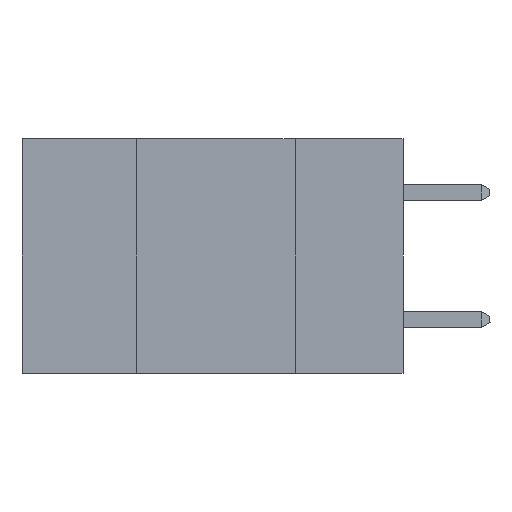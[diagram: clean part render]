
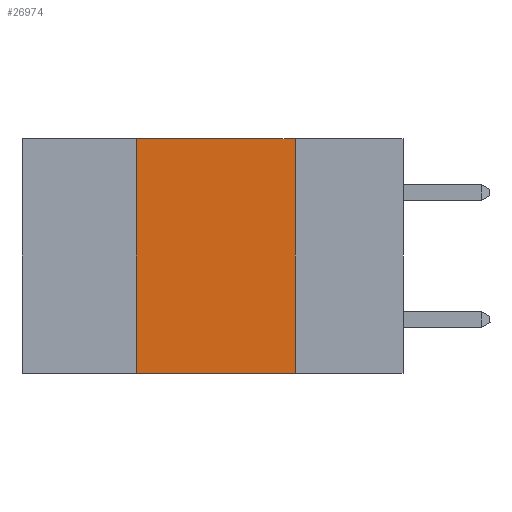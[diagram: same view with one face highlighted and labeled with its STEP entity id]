
A CAD part, left-side view. The second image highlights one B-rep face of the part: STEP entity #26974.
In plain terms, the highlighted planar face has unit normal (-1, 0, 0).
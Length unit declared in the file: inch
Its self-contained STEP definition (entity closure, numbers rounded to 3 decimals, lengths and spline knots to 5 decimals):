
#335 = CARTESIAN_POINT ( 'NONE',  ( 0., 0.6, -0.37 ) ) ;
#423 = EDGE_LOOP ( 'NONE', ( #12382, #18874, #16290, #22187 ) ) ;
#1531 = CARTESIAN_POINT ( 'NONE',  ( 0., 0.42, 0. ) ) ;
#4603 = CARTESIAN_POINT ( 'NONE',  ( 0., 0.17, -0.37 ) ) ;
#5061 = VERTEX_POINT ( 'NONE', #4603 ) ;
#5590 = EDGE_CURVE ( 'NONE', #26018, #29388, #32946, .T. ) ;
#6365 = PLANE ( 'NONE',  #26450 ) ;
#6553 = DIRECTION ( 'NONE',  ( 0., 0., 1. ) ) ;
#7317 = VECTOR ( 'NONE', #6553, 39.37008 ) ;
#8792 = FACE_OUTER_BOUND ( 'NONE', #423, .T. ) ;
#8803 = CARTESIAN_POINT ( 'NONE',  ( 0., 0.42, 0. ) ) ;
#9530 = DIRECTION ( 'NONE',  ( 0., -1., 0. ) ) ;
#9586 = EDGE_CURVE ( 'NONE', #29388, #25753, #22335, .T. ) ;
#10875 = LINE ( 'NONE', #335, #19131 ) ;
#11165 = VECTOR ( 'NONE', #9530, 39.37008 ) ;
#11464 = CARTESIAN_POINT ( 'NONE',  ( 0., 0.6, 0. ) ) ;
#12179 = LINE ( 'NONE', #23573, #29580 ) ;
#12382 = ORIENTED_EDGE ( 'NONE', *, *, #25512, .F. ) ;
#15011 = CARTESIAN_POINT ( 'NONE',  ( 0., 0.6, 0. ) ) ;
#16290 = ORIENTED_EDGE ( 'NONE', *, *, #5590, .F. ) ;
#18395 = DIRECTION ( 'NONE',  ( 0., -1., 0. ) ) ;
#18874 = ORIENTED_EDGE ( 'NONE', *, *, #9586, .F. ) ;
#19131 = VECTOR ( 'NONE', #18395, 39.37008 ) ;
#22176 = CARTESIAN_POINT ( 'NONE',  ( 0., 0.17, 0. ) ) ;
#22187 = ORIENTED_EDGE ( 'NONE', *, *, #32123, .T. ) ;
#22335 = LINE ( 'NONE', #15011, #11165 ) ;
#23573 = CARTESIAN_POINT ( 'NONE',  ( 0., 0.17, 0. ) ) ;
#24887 = DIRECTION ( 'NONE',  ( 0., 0., -1. ) ) ;
#25512 = EDGE_CURVE ( 'NONE', #25753, #5061, #12179, .T. ) ;
#25753 = VERTEX_POINT ( 'NONE', #22176 ) ;
#26018 = VERTEX_POINT ( 'NONE', #33610 ) ;
#26450 = AXIS2_PLACEMENT_3D ( 'NONE', #11464, #32633, #24887 ) ;
#26974 = ADVANCED_FACE ( 'NONE', ( #8792 ), #6365, .F. ) ;
#29388 = VERTEX_POINT ( 'NONE', #1531 ) ;
#29580 = VECTOR ( 'NONE', #31633, 39.37008 ) ;
#31633 = DIRECTION ( 'NONE',  ( 0., 0., -1. ) ) ;
#32123 = EDGE_CURVE ( 'NONE', #26018, #5061, #10875, .T. ) ;
#32633 = DIRECTION ( 'NONE',  ( 1., 0., 0. ) ) ;
#32946 = LINE ( 'NONE', #8803, #7317 ) ;
#33610 = CARTESIAN_POINT ( 'NONE',  ( 0., 0.42, -0.37 ) ) ;
